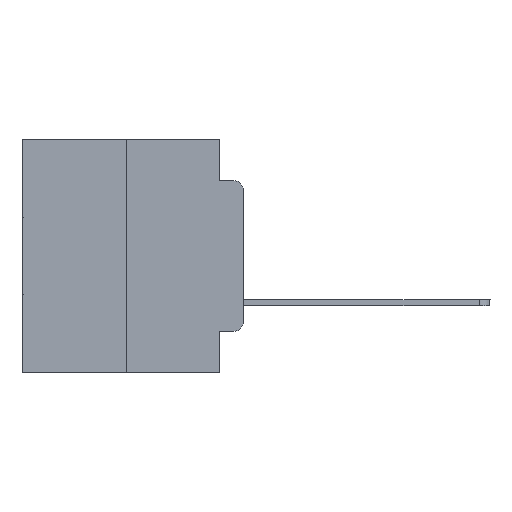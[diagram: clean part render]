
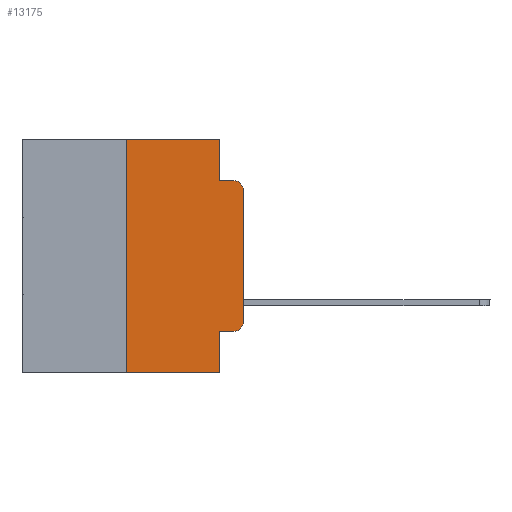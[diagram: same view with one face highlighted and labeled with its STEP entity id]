
A CAD part, left-side view. The second image highlights one B-rep face of the part: STEP entity #13175.
In plain terms, the highlighted planar face has unit normal (-1, 0, 0).
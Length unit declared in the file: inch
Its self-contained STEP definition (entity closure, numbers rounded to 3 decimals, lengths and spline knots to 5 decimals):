
#32 = ORIENTED_EDGE ( 'NONE', *, *, #3641, .F. ) ;
#457 = LINE ( 'NONE', #22003, #17241 ) ;
#1031 = EDGE_CURVE ( 'NONE', #22688, #14238, #14429, .T. ) ;
#1396 = DIRECTION ( 'NONE',  ( -1., 0., 0. ) ) ;
#1729 = EDGE_LOOP ( 'NONE', ( #10946, #22504, #13344, #22658, #23203, #32, #18195, #7968, #6311, #6935 ) ) ;
#1730 = LINE ( 'NONE', #13162, #4809 ) ;
#1828 = DIRECTION ( 'NONE',  ( 0., 0., -1. ) ) ;
#2454 = CARTESIAN_POINT ( 'NONE',  ( 0., 0.25, -0.5 ) ) ;
#2876 = DIRECTION ( 'NONE',  ( 0., -1., 0. ) ) ;
#2942 = VERTEX_POINT ( 'NONE', #19959 ) ;
#3310 = VERTEX_POINT ( 'NONE', #14369 ) ;
#3641 = EDGE_CURVE ( 'NONE', #22753, #6990, #4969, .T. ) ;
#4367 = VECTOR ( 'NONE', #17423, 39.37008 ) ;
#4411 = CARTESIAN_POINT ( 'NONE',  ( 0., 0., 0. ) ) ;
#4420 = VECTOR ( 'NONE', #15484, 39.37008 ) ;
#4809 = VECTOR ( 'NONE', #17529, 39.37008 ) ;
#4969 = LINE ( 'NONE', #11107, #27569 ) ;
#5494 = CARTESIAN_POINT ( 'NONE',  ( 0., 0.25, 0. ) ) ;
#5885 = EDGE_CURVE ( 'NONE', #3310, #15705, #14885, .T. ) ;
#6311 = ORIENTED_EDGE ( 'NONE', *, *, #6707, .T. ) ;
#6707 = EDGE_CURVE ( 'NONE', #20068, #22688, #457, .T. ) ;
#6935 = ORIENTED_EDGE ( 'NONE', *, *, #1031, .T. ) ;
#6990 = VERTEX_POINT ( 'NONE', #5494 ) ;
#7093 = FACE_OUTER_BOUND ( 'NONE', #1729, .T. ) ;
#7735 = CARTESIAN_POINT ( 'NONE',  ( 0., 0.051, 0. ) ) ;
#7968 = ORIENTED_EDGE ( 'NONE', *, *, #13793, .F. ) ;
#8201 = CARTESIAN_POINT ( 'NONE',  ( 0., 0.051, -0.0885 ) ) ;
#8794 = DIRECTION ( 'NONE',  ( 0., 0., -1. ) ) ;
#9768 = VECTOR ( 'NONE', #2876, 39.37008 ) ;
#10893 = AXIS2_PLACEMENT_3D ( 'NONE', #25560, #21354, #23280 ) ;
#10946 = ORIENTED_EDGE ( 'NONE', *, *, #13263, .T. ) ;
#11107 = CARTESIAN_POINT ( 'NONE',  ( 0., 0.25, 0. ) ) ;
#11407 = CARTESIAN_POINT ( 'NONE',  ( 0., 0.051, -0.4115 ) ) ;
#12101 = EDGE_CURVE ( 'NONE', #18377, #3310, #25646, .T. ) ;
#12884 = DIRECTION ( 'NONE',  ( 0., -1., 0. ) ) ;
#13162 = CARTESIAN_POINT ( 'NONE',  ( 0., 0.473, 0. ) ) ;
#13175 = ADVANCED_FACE ( 'NONE', ( #7093 ), #18941, .F. ) ;
#13263 = EDGE_CURVE ( 'NONE', #14238, #2942, #23916, .T. ) ;
#13344 = ORIENTED_EDGE ( 'NONE', *, *, #5885, .F. ) ;
#13480 = VECTOR ( 'NONE', #12884, 39.37008 ) ;
#13793 = EDGE_CURVE ( 'NONE', #20068, #23833, #27269, .T. ) ;
#14238 = VERTEX_POINT ( 'NONE', #15207 ) ;
#14369 = CARTESIAN_POINT ( 'NONE',  ( 0., 0.051, -0.0885 ) ) ;
#14429 = CIRCLE ( 'NONE', #18116, 0.02 ) ;
#14885 = LINE ( 'NONE', #8201, #9768 ) ;
#15207 = CARTESIAN_POINT ( 'NONE',  ( 0., 0., -0.3915 ) ) ;
#15484 = DIRECTION ( 'NONE',  ( 0., 0., -1. ) ) ;
#15535 = LINE ( 'NONE', #19634, #13480 ) ;
#15569 = DIRECTION ( 'NONE',  ( -1., 0., 0. ) ) ;
#15705 = VERTEX_POINT ( 'NONE', #25538 ) ;
#17126 = CARTESIAN_POINT ( 'NONE',  ( 0., 0.051, -0.5 ) ) ;
#17241 = VECTOR ( 'NONE', #17296, 39.37008 ) ;
#17296 = DIRECTION ( 'NONE',  ( 0., -1., 0. ) ) ;
#17423 = DIRECTION ( 'NONE',  ( 0., 0., 1. ) ) ;
#17529 = DIRECTION ( 'NONE',  ( 0., -1., 0. ) ) ;
#17558 = CARTESIAN_POINT ( 'NONE',  ( 0., 0.02, -0.4115 ) ) ;
#18116 = AXIS2_PLACEMENT_3D ( 'NONE', #27809, #1396, #25610 ) ;
#18195 = ORIENTED_EDGE ( 'NONE', *, *, #23351, .T. ) ;
#18377 = VERTEX_POINT ( 'NONE', #19608 ) ;
#18941 = PLANE ( 'NONE',  #10893 ) ;
#19376 = VECTOR ( 'NONE', #1828, 39.37008 ) ;
#19608 = CARTESIAN_POINT ( 'NONE',  ( 0., 0.051, 0. ) ) ;
#19634 = CARTESIAN_POINT ( 'NONE',  ( 0., 0.473, -0.5 ) ) ;
#19951 = CARTESIAN_POINT ( 'NONE',  ( 0., 0.02, -0.1085 ) ) ;
#19959 = CARTESIAN_POINT ( 'NONE',  ( 0., 0., -0.1085 ) ) ;
#20068 = VERTEX_POINT ( 'NONE', #11407 ) ;
#20142 = AXIS2_PLACEMENT_3D ( 'NONE', #19951, #15569, #8794 ) ;
#20441 = DIRECTION ( 'NONE',  ( 0., 0., 1. ) ) ;
#21354 = DIRECTION ( 'NONE',  ( 1., 0., 0. ) ) ;
#22003 = CARTESIAN_POINT ( 'NONE',  ( 0., 0.051, -0.4115 ) ) ;
#22504 = ORIENTED_EDGE ( 'NONE', *, *, #22709, .T. ) ;
#22658 = ORIENTED_EDGE ( 'NONE', *, *, #12101, .F. ) ;
#22688 = VERTEX_POINT ( 'NONE', #17558 ) ;
#22709 = EDGE_CURVE ( 'NONE', #2942, #15705, #25139, .T. ) ;
#22753 = VERTEX_POINT ( 'NONE', #2454 ) ;
#23203 = ORIENTED_EDGE ( 'NONE', *, *, #25978, .F. ) ;
#23280 = DIRECTION ( 'NONE',  ( 0., 0., -1. ) ) ;
#23351 = EDGE_CURVE ( 'NONE', #22753, #23833, #15535, .T. ) ;
#23833 = VERTEX_POINT ( 'NONE', #17126 ) ;
#23916 = LINE ( 'NONE', #4411, #4367 ) ;
#25139 = CIRCLE ( 'NONE', #20142, 0.02 ) ;
#25538 = CARTESIAN_POINT ( 'NONE',  ( 0., 0.02, -0.0885 ) ) ;
#25560 = CARTESIAN_POINT ( 'NONE',  ( 0., 0.473, 0. ) ) ;
#25610 = DIRECTION ( 'NONE',  ( 0., 0., -1. ) ) ;
#25646 = LINE ( 'NONE', #7735, #4420 ) ;
#25978 = EDGE_CURVE ( 'NONE', #6990, #18377, #1730, .T. ) ;
#27269 = LINE ( 'NONE', #27300, #19376 ) ;
#27300 = CARTESIAN_POINT ( 'NONE',  ( 0., 0.051, 0. ) ) ;
#27569 = VECTOR ( 'NONE', #20441, 39.37008 ) ;
#27809 = CARTESIAN_POINT ( 'NONE',  ( 0., 0.02, -0.3915 ) ) ;
